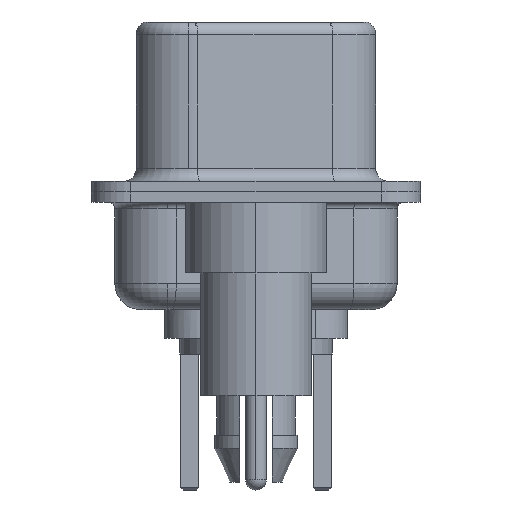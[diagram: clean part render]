
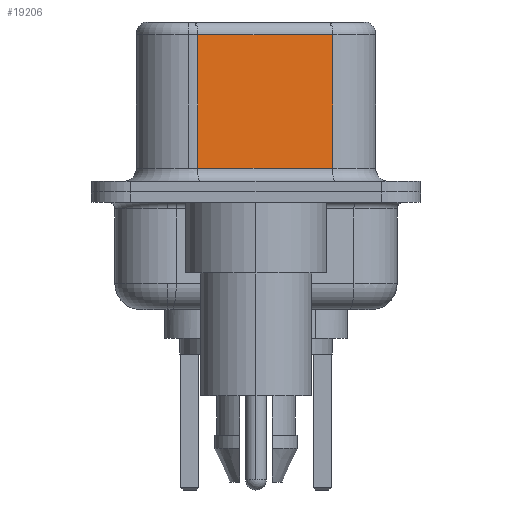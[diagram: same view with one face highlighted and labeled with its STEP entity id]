
A CAD part, left-side view. The second image highlights one B-rep face of the part: STEP entity #19206.
In plain terms, the highlighted planar face has unit normal (-0.985, -0.174, 0).
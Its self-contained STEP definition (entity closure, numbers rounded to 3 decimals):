
#237 = EDGE_CURVE ( 'NONE', #18710, #12998, #14888, .T. ) ;
#874 = PLANE ( 'NONE',  #11965 ) ;
#1489 = LINE ( 'NONE', #7498, #8607 ) ;
#1722 = DIRECTION ( 'NONE',  ( 0.174, -0.985, 0. ) ) ;
#2150 = CARTESIAN_POINT ( 'NONE',  ( 3.67, 2.233, 6.02 ) ) ;
#3439 = DIRECTION ( 'NONE',  ( -0.174, 0.985, 0. ) ) ;
#3540 = VECTOR ( 'NONE', #3439, 1000. ) ;
#3767 = CARTESIAN_POINT ( 'NONE',  ( 3.67, 2.233, 0.9 ) ) ;
#4189 = ORIENTED_EDGE ( 'NONE', *, *, #237, .T. ) ;
#5368 = CARTESIAN_POINT ( 'NONE',  ( 4.58, -2.927, 0.9 ) ) ;
#6752 = FACE_OUTER_BOUND ( 'NONE', #20356, .T. ) ;
#7191 = ORIENTED_EDGE ( 'NONE', *, *, #17602, .F. ) ;
#7498 = CARTESIAN_POINT ( 'NONE',  ( 3.67, 2.233, 6.52 ) ) ;
#7538 = DIRECTION ( 'NONE',  ( 0., 0., -1. ) ) ;
#8543 = EDGE_CURVE ( 'NONE', #16899, #18710, #1489, .T. ) ;
#8607 = VECTOR ( 'NONE', #13093, 1000. ) ;
#9959 = LINE ( 'NONE', #16769, #22626 ) ;
#11871 = DIRECTION ( 'NONE',  ( 0.985, 0.174, 0. ) ) ;
#11965 = AXIS2_PLACEMENT_3D ( 'NONE', #13552, #11871, #19023 ) ;
#12998 = VERTEX_POINT ( 'NONE', #15878 ) ;
#13093 = DIRECTION ( 'NONE',  ( 0., 0., -1. ) ) ;
#13260 = LINE ( 'NONE', #20130, #3540 ) ;
#13552 = CARTESIAN_POINT ( 'NONE',  ( 4.58, -2.927, 6.52 ) ) ;
#14888 = LINE ( 'NONE', #5368, #16031 ) ;
#15878 = CARTESIAN_POINT ( 'NONE',  ( 4.58, -2.927, 0.9 ) ) ;
#16031 = VECTOR ( 'NONE', #1722, 1000. ) ;
#16442 = VERTEX_POINT ( 'NONE', #22681 ) ;
#16769 = CARTESIAN_POINT ( 'NONE',  ( 4.58, -2.927, 6.52 ) ) ;
#16899 = VERTEX_POINT ( 'NONE', #2150 ) ;
#17602 = EDGE_CURVE ( 'NONE', #16442, #12998, #9959, .T. ) ;
#18710 = VERTEX_POINT ( 'NONE', #3767 ) ;
#19023 = DIRECTION ( 'NONE',  ( -0.174, 0.985, 0. ) ) ;
#19206 = ADVANCED_FACE ( 'NONE', ( #6752 ), #874, .F. ) ;
#19892 = ORIENTED_EDGE ( 'NONE', *, *, #21291, .T. ) ;
#20130 = CARTESIAN_POINT ( 'NONE',  ( 4.58, -2.927, 6.02 ) ) ;
#20356 = EDGE_LOOP ( 'NONE', ( #7191, #19892, #21161, #4189 ) ) ;
#21161 = ORIENTED_EDGE ( 'NONE', *, *, #8543, .T. ) ;
#21291 = EDGE_CURVE ( 'NONE', #16442, #16899, #13260, .T. ) ;
#22626 = VECTOR ( 'NONE', #7538, 1000. ) ;
#22681 = CARTESIAN_POINT ( 'NONE',  ( 4.58, -2.927, 6.02 ) ) ;
